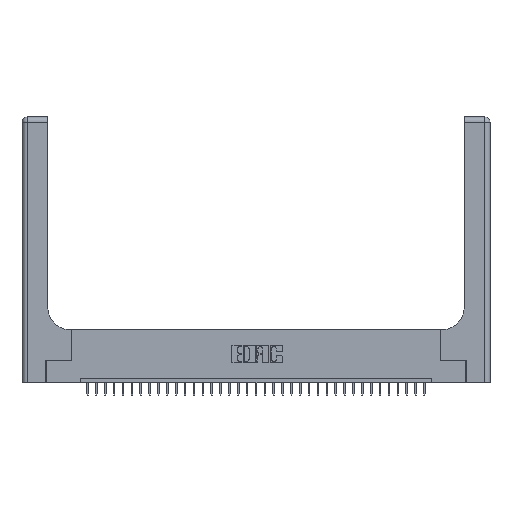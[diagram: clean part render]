
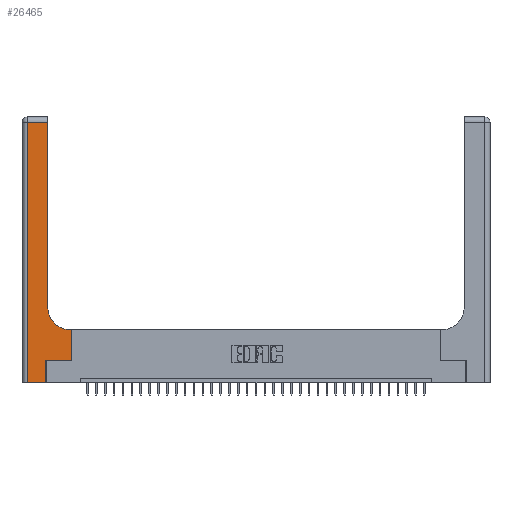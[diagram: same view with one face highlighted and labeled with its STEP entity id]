
A CAD part, top view. The second image highlights one B-rep face of the part: STEP entity #26465.
In plain terms, the highlighted planar face has unit normal (0, 0, 1).
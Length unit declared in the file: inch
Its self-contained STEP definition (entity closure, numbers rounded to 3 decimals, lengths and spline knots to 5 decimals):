
#327 = VECTOR ( 'NONE', #22026, 39.37008 ) ;
#390 = LINE ( 'NONE', #11206, #327 ) ;
#809 = DIRECTION ( 'NONE',  ( 0., 1., 0. ) ) ;
#1465 = ORIENTED_EDGE ( 'NONE', *, *, #14416, .T. ) ;
#2181 = CARTESIAN_POINT ( 'NONE',  ( 0.06, 2.94, 0.37 ) ) ;
#2577 = VECTOR ( 'NONE', #809, 39.37008 ) ;
#2894 = LINE ( 'NONE', #30166, #4711 ) ;
#3143 = CARTESIAN_POINT ( 'NONE',  ( 0.269, 0., 0.37 ) ) ;
#3238 = EDGE_CURVE ( 'NONE', #13184, #15955, #2894, .T. ) ;
#3479 = EDGE_CURVE ( 'NONE', #21669, #16638, #23291, .T. ) ;
#3509 = CARTESIAN_POINT ( 'NONE',  ( 0.5415, 0.6, 0.37 ) ) ;
#4291 = DIRECTION ( 'NONE',  ( 1., 0., 0. ) ) ;
#4711 = VECTOR ( 'NONE', #5922, 39.37008 ) ;
#5128 = EDGE_LOOP ( 'NONE', ( #25284, #11208, #18488, #1465, #6172, #6238, #34408, #23588, #13163 ) ) ;
#5922 = DIRECTION ( 'NONE',  ( -1., 0., 0. ) ) ;
#6172 = ORIENTED_EDGE ( 'NONE', *, *, #30165, .T. ) ;
#6238 = ORIENTED_EDGE ( 'NONE', *, *, #3479, .T. ) ;
#7496 = VECTOR ( 'NONE', #22459, 39.37008 ) ;
#8417 = CARTESIAN_POINT ( 'NONE',  ( 0.2915, 3., 0.37 ) ) ;
#8469 = DIRECTION ( 'NONE',  ( 0., 1., 0. ) ) ;
#8966 = CARTESIAN_POINT ( 'NONE',  ( 0.5585, 0.25, 0.37 ) ) ;
#10096 = CARTESIAN_POINT ( 'NONE',  ( 0.5585, 0.6, 0.37 ) ) ;
#11076 = LINE ( 'NONE', #8417, #19623 ) ;
#11206 = CARTESIAN_POINT ( 'NONE',  ( 0.06, 3., 0.37 ) ) ;
#11208 = ORIENTED_EDGE ( 'NONE', *, *, #21576, .T. ) ;
#11514 = CARTESIAN_POINT ( 'NONE',  ( 0., 0., 0.37 ) ) ;
#11644 = EDGE_CURVE ( 'NONE', #16638, #13184, #25100, .T. ) ;
#13163 = ORIENTED_EDGE ( 'NONE', *, *, #19667, .T. ) ;
#13184 = VERTEX_POINT ( 'NONE', #10096 ) ;
#13688 = CARTESIAN_POINT ( 'NONE',  ( 0.5585, 0.25, 0.37 ) ) ;
#14055 = FACE_OUTER_BOUND ( 'NONE', #5128, .T. ) ;
#14245 = DIRECTION ( 'NONE',  ( 0., 1., 0. ) ) ;
#14416 = EDGE_CURVE ( 'NONE', #16374, #24037, #17012, .T. ) ;
#15453 = CARTESIAN_POINT ( 'NONE',  ( 0.2915, 2.94, 0.37 ) ) ;
#15955 = VERTEX_POINT ( 'NONE', #3509 ) ;
#16374 = VERTEX_POINT ( 'NONE', #27400 ) ;
#16638 = VERTEX_POINT ( 'NONE', #13688 ) ;
#17012 = LINE ( 'NONE', #11514, #25864 ) ;
#17149 = LINE ( 'NONE', #3143, #21360 ) ;
#18488 = ORIENTED_EDGE ( 'NONE', *, *, #28225, .T. ) ;
#19389 = VECTOR ( 'NONE', #23455, 39.37008 ) ;
#19574 = VERTEX_POINT ( 'NONE', #15453 ) ;
#19623 = VECTOR ( 'NONE', #14245, 39.37008 ) ;
#19667 = EDGE_CURVE ( 'NONE', #15955, #26185, #34515, .T. ) ;
#19791 = CARTESIAN_POINT ( 'NONE',  ( 0.269, 0., 0.37 ) ) ;
#20422 = DIRECTION ( 'NONE',  ( 0., 0., -1. ) ) ;
#20618 = CARTESIAN_POINT ( 'NONE',  ( 0.269, 0.25, 0.37 ) ) ;
#21360 = VECTOR ( 'NONE', #8469, 39.37008 ) ;
#21576 = EDGE_CURVE ( 'NONE', #19574, #24670, #24936, .T. ) ;
#21669 = VERTEX_POINT ( 'NONE', #30744 ) ;
#22026 = DIRECTION ( 'NONE',  ( 0., -1., 0. ) ) ;
#22243 = CARTESIAN_POINT ( 'NONE',  ( 0., 3., 0.37 ) ) ;
#22356 = DIRECTION ( 'NONE',  ( 1., 0., 0. ) ) ;
#22459 = DIRECTION ( 'NONE',  ( -1., 0., 0. ) ) ;
#23291 = LINE ( 'NONE', #20618, #19389 ) ;
#23455 = DIRECTION ( 'NONE',  ( 1., 0., 0. ) ) ;
#23588 = ORIENTED_EDGE ( 'NONE', *, *, #3238, .T. ) ;
#24037 = VERTEX_POINT ( 'NONE', #19791 ) ;
#24670 = VERTEX_POINT ( 'NONE', #2181 ) ;
#24903 = PLANE ( 'NONE',  #28556 ) ;
#24936 = LINE ( 'NONE', #25109, #7496 ) ;
#25100 = LINE ( 'NONE', #8966, #2577 ) ;
#25109 = CARTESIAN_POINT ( 'NONE',  ( 0., 2.94, 0.37 ) ) ;
#25284 = ORIENTED_EDGE ( 'NONE', *, *, #29442, .T. ) ;
#25864 = VECTOR ( 'NONE', #22356, 39.37008 ) ;
#26185 = VERTEX_POINT ( 'NONE', #29170 ) ;
#26465 = ADVANCED_FACE ( 'NONE', ( #14055 ), #24903, .F. ) ;
#27400 = CARTESIAN_POINT ( 'NONE',  ( 0.06, 0., 0.37 ) ) ;
#28225 = EDGE_CURVE ( 'NONE', #24670, #16374, #390, .T. ) ;
#28556 = AXIS2_PLACEMENT_3D ( 'NONE', #22243, #33017, #33212 ) ;
#29170 = CARTESIAN_POINT ( 'NONE',  ( 0.2915, 0.85, 0.37 ) ) ;
#29442 = EDGE_CURVE ( 'NONE', #26185, #19574, #11076, .T. ) ;
#30165 = EDGE_CURVE ( 'NONE', #24037, #21669, #17149, .T. ) ;
#30166 = CARTESIAN_POINT ( 'NONE',  ( 0.2915, 0.6, 0.37 ) ) ;
#30744 = CARTESIAN_POINT ( 'NONE',  ( 0.269, 0.25, 0.37 ) ) ;
#33017 = DIRECTION ( 'NONE',  ( 0., 0., -1. ) ) ;
#33212 = DIRECTION ( 'NONE',  ( -1., 0., 0. ) ) ;
#33891 = CARTESIAN_POINT ( 'NONE',  ( 0.5415, 0.85, 0.37 ) ) ;
#33934 = AXIS2_PLACEMENT_3D ( 'NONE', #33891, #20422, #4291 ) ;
#34408 = ORIENTED_EDGE ( 'NONE', *, *, #11644, .T. ) ;
#34515 = CIRCLE ( 'NONE', #33934, 0.25 ) ;
